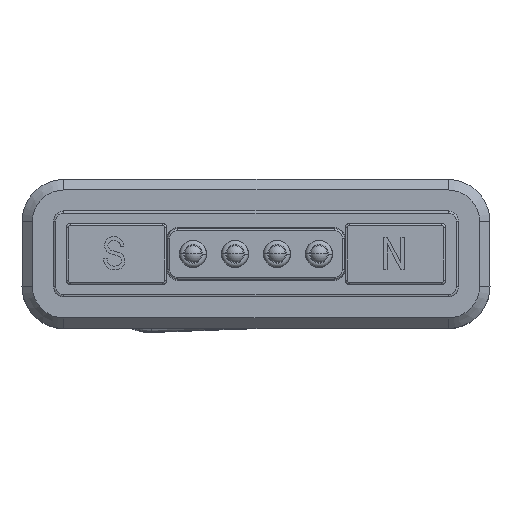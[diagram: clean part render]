
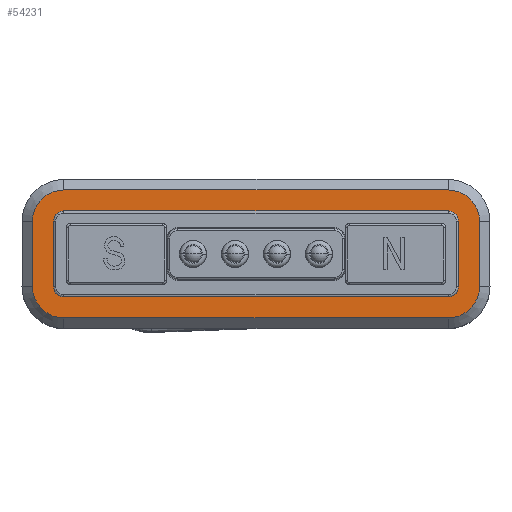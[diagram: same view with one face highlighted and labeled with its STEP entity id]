
A CAD part, top view. The second image highlights one B-rep face of the part: STEP entity #54231.
In plain terms, the highlighted planar face has unit normal (0, 0, 1).
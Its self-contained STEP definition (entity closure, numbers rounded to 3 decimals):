
#741 = AXIS2_PLACEMENT_3D ( 'NONE', #9683, #37258, #10805 ) ;
#1030 = CARTESIAN_POINT ( 'NONE',  ( -10.65, -1.55, -0.5 ) ) ;
#1350 = ORIENTED_EDGE ( 'NONE', *, *, #19401, .F. ) ;
#1521 = DIRECTION ( 'NONE',  ( 0., 0., -1. ) ) ;
#2647 = DIRECTION ( 'NONE',  ( 0., 1., 0. ) ) ;
#2835 = ORIENTED_EDGE ( 'NONE', *, *, #43955, .T. ) ;
#3294 = EDGE_CURVE ( 'NONE', #37424, #54211, #42026, .T. ) ;
#3848 = CIRCLE ( 'NONE', #7521, 1.5 ) ;
#4217 = VECTOR ( 'NONE', #20566, 1000. ) ;
#5425 = CARTESIAN_POINT ( 'NONE',  ( -9.65, -1.55, -0.5 ) ) ;
#5600 = DIRECTION ( 'NONE',  ( 0., 1., 0. ) ) ;
#5861 = DIRECTION ( 'NONE',  ( 0., 0., -1. ) ) ;
#5863 = VERTEX_POINT ( 'NONE', #23645 ) ;
#6089 = DIRECTION ( 'NONE',  ( 0., 0., -1. ) ) ;
#6376 = CARTESIAN_POINT ( 'NONE',  ( 9.15, -1.55, -0.5 ) ) ;
#6567 = ORIENTED_EDGE ( 'NONE', *, *, #45096, .F. ) ;
#6607 = VERTEX_POINT ( 'NONE', #5425 ) ;
#6695 = CIRCLE ( 'NONE', #25925, 0.5 ) ;
#6750 = CIRCLE ( 'NONE', #46231, 0.5 ) ;
#6774 = CIRCLE ( 'NONE', #22342, 1.5 ) ;
#7424 = CARTESIAN_POINT ( 'NONE',  ( -9.15, 3.05, -0.5 ) ) ;
#7521 = AXIS2_PLACEMENT_3D ( 'NONE', #19333, #36062, #5600 ) ;
#8927 = LINE ( 'NONE', #26409, #50702 ) ;
#9656 = CARTESIAN_POINT ( 'NONE',  ( -9.15, -2.05, -0.5 ) ) ;
#9683 = CARTESIAN_POINT ( 'NONE',  ( 0., 0., -0.5 ) ) ;
#10805 = DIRECTION ( 'NONE',  ( 1., 0., 0. ) ) ;
#11178 = DIRECTION ( 'NONE',  ( 0., -1., 0. ) ) ;
#11232 = EDGE_CURVE ( 'NONE', #11741, #42800, #41487, .T. ) ;
#11365 = CARTESIAN_POINT ( 'NONE',  ( 10.65, 1.55, -0.5 ) ) ;
#11433 = DIRECTION ( 'NONE',  ( 1., 0., 0. ) ) ;
#11741 = VERTEX_POINT ( 'NONE', #11365 ) ;
#11867 = DIRECTION ( 'NONE',  ( 0., 0., 1. ) ) ;
#12131 = AXIS2_PLACEMENT_3D ( 'NONE', #43207, #11867, #51248 ) ;
#12845 = VECTOR ( 'NONE', #36100, 1000. ) ;
#12846 = CARTESIAN_POINT ( 'NONE',  ( 9.15, -3.05, -0.5 ) ) ;
#12920 = ORIENTED_EDGE ( 'NONE', *, *, #42680, .T. ) ;
#12980 = CARTESIAN_POINT ( 'NONE',  ( -10.65, 1.55, -0.5 ) ) ;
#14417 = EDGE_CURVE ( 'NONE', #39064, #35145, #6750, .T. ) ;
#14710 = DIRECTION ( 'NONE',  ( -1., 0., 0. ) ) ;
#15049 = CIRCLE ( 'NONE', #26985, 0.5 ) ;
#15446 = LINE ( 'NONE', #51396, #35349 ) ;
#15477 = DIRECTION ( 'NONE',  ( 0., 0., 1. ) ) ;
#15517 = ORIENTED_EDGE ( 'NONE', *, *, #45349, .F. ) ;
#16458 = CARTESIAN_POINT ( 'NONE',  ( 9.15, 3.05, -0.5 ) ) ;
#16948 = DIRECTION ( 'NONE',  ( 0., -1., 0. ) ) ;
#16965 = VECTOR ( 'NONE', #43349, 1000. ) ;
#17939 = AXIS2_PLACEMENT_3D ( 'NONE', #40098, #5861, #27656 ) ;
#18100 = DIRECTION ( 'NONE',  ( -1., 0., 0. ) ) ;
#18328 = EDGE_LOOP ( 'NONE', ( #38152, #49532, #15517, #2835, #1350, #30088, #6567, #12920 ) ) ;
#18945 = CARTESIAN_POINT ( 'NONE',  ( -9.15, -2.05, -0.5 ) ) ;
#19059 = AXIS2_PLACEMENT_3D ( 'NONE', #26972, #45114, #18100 ) ;
#19333 = CARTESIAN_POINT ( 'NONE',  ( -9.15, 1.55, -0.5 ) ) ;
#19401 = EDGE_CURVE ( 'NONE', #11741, #5863, #43627, .T. ) ;
#19485 = VERTEX_POINT ( 'NONE', #39598 ) ;
#20566 = DIRECTION ( 'NONE',  ( 0., -1., 0. ) ) ;
#21087 = CARTESIAN_POINT ( 'NONE',  ( -9.15, 2.05, -0.5 ) ) ;
#21243 = EDGE_LOOP ( 'NONE', ( #50930, #36769, #32887, #30159, #35294, #39664, #36123, #38819 ) ) ;
#22342 = AXIS2_PLACEMENT_3D ( 'NONE', #54898, #15477, #11178 ) ;
#22556 = PLANE ( 'NONE',  #741 ) ;
#22831 = FACE_OUTER_BOUND ( 'NONE', #18328, .T. ) ;
#23645 = CARTESIAN_POINT ( 'NONE',  ( 10.65, -1.55, -0.5 ) ) ;
#23890 = CARTESIAN_POINT ( 'NONE',  ( -9.15, -3.05, -0.5 ) ) ;
#24522 = EDGE_CURVE ( 'NONE', #39064, #6607, #25183, .T. ) ;
#25183 = LINE ( 'NONE', #55174, #42379 ) ;
#25925 = AXIS2_PLACEMENT_3D ( 'NONE', #6376, #1521, #30615 ) ;
#26409 = CARTESIAN_POINT ( 'NONE',  ( -10.65, 1.55, -0.5 ) ) ;
#26413 = EDGE_CURVE ( 'NONE', #19485, #35145, #46057, .T. ) ;
#26972 = CARTESIAN_POINT ( 'NONE',  ( -9.15, -1.55, -0.5 ) ) ;
#26985 = AXIS2_PLACEMENT_3D ( 'NONE', #45451, #6089, #31964 ) ;
#27656 = DIRECTION ( 'NONE',  ( 0., 1., 0. ) ) ;
#29345 = DIRECTION ( 'NONE',  ( 0., 0., -1. ) ) ;
#29415 = EDGE_CURVE ( 'NONE', #35262, #46931, #55821, .T. ) ;
#30088 = ORIENTED_EDGE ( 'NONE', *, *, #11232, .T. ) ;
#30159 = ORIENTED_EDGE ( 'NONE', *, *, #26413, .F. ) ;
#30483 = CARTESIAN_POINT ( 'NONE',  ( 9.65, -1.55, -0.5 ) ) ;
#30615 = DIRECTION ( 'NONE',  ( 1., 0., 0. ) ) ;
#31964 = DIRECTION ( 'NONE',  ( 0., -1., 0. ) ) ;
#32887 = ORIENTED_EDGE ( 'NONE', *, *, #14417, .T. ) ;
#33658 = VECTOR ( 'NONE', #2647, 1000. ) ;
#33937 = CARTESIAN_POINT ( 'NONE',  ( 9.15, -3.05, -0.5 ) ) ;
#34434 = LINE ( 'NONE', #12846, #16965 ) ;
#35145 = VERTEX_POINT ( 'NONE', #21087 ) ;
#35262 = VERTEX_POINT ( 'NONE', #1030 ) ;
#35294 = ORIENTED_EDGE ( 'NONE', *, *, #45796, .T. ) ;
#35349 = VECTOR ( 'NONE', #11433, 1000. ) ;
#35568 = CARTESIAN_POINT ( 'NONE',  ( 9.65, 1.55, -0.5 ) ) ;
#36062 = DIRECTION ( 'NONE',  ( 0., 0., 1. ) ) ;
#36100 = DIRECTION ( 'NONE',  ( 1., 0., 0. ) ) ;
#36123 = ORIENTED_EDGE ( 'NONE', *, *, #43632, .T. ) ;
#36769 = ORIENTED_EDGE ( 'NONE', *, *, #24522, .F. ) ;
#37258 = DIRECTION ( 'NONE',  ( 0., 0., 1. ) ) ;
#37424 = VERTEX_POINT ( 'NONE', #30483 ) ;
#38152 = ORIENTED_EDGE ( 'NONE', *, *, #43210, .T. ) ;
#38358 = VERTEX_POINT ( 'NONE', #18945 ) ;
#38819 = ORIENTED_EDGE ( 'NONE', *, *, #40412, .F. ) ;
#39064 = VERTEX_POINT ( 'NONE', #41227 ) ;
#39327 = CARTESIAN_POINT ( 'NONE',  ( 10.65, 1.55, -0.5 ) ) ;
#39598 = CARTESIAN_POINT ( 'NONE',  ( 9.15, 2.05, -0.5 ) ) ;
#39664 = ORIENTED_EDGE ( 'NONE', *, *, #3294, .F. ) ;
#39927 = VERTEX_POINT ( 'NONE', #33937 ) ;
#40098 = CARTESIAN_POINT ( 'NONE',  ( 9.15, 1.55, -0.5 ) ) ;
#40412 = EDGE_CURVE ( 'NONE', #38358, #52017, #49038, .T. ) ;
#40767 = VERTEX_POINT ( 'NONE', #12980 ) ;
#41227 = CARTESIAN_POINT ( 'NONE',  ( -9.65, 1.55, -0.5 ) ) ;
#41487 = CIRCLE ( 'NONE', #12131, 1.5 ) ;
#42026 = LINE ( 'NONE', #45460, #33658 ) ;
#42379 = VECTOR ( 'NONE', #56020, 1000. ) ;
#42680 = EDGE_CURVE ( 'NONE', #45193, #40767, #3848, .T. ) ;
#42770 = CIRCLE ( 'NONE', #17939, 0.5 ) ;
#42800 = VERTEX_POINT ( 'NONE', #16458 ) ;
#43207 = CARTESIAN_POINT ( 'NONE',  ( 9.15, 1.55, -0.5 ) ) ;
#43210 = EDGE_CURVE ( 'NONE', #40767, #35262, #8927, .T. ) ;
#43349 = DIRECTION ( 'NONE',  ( -1., 0., 0. ) ) ;
#43627 = LINE ( 'NONE', #39327, #4217 ) ;
#43632 = EDGE_CURVE ( 'NONE', #37424, #52017, #6695, .T. ) ;
#43954 = CARTESIAN_POINT ( 'NONE',  ( 9.15, -2.05, -0.5 ) ) ;
#43955 = EDGE_CURVE ( 'NONE', #39927, #5863, #6774, .T. ) ;
#45096 = EDGE_CURVE ( 'NONE', #45193, #42800, #15446, .T. ) ;
#45114 = DIRECTION ( 'NONE',  ( 0., 0., 1. ) ) ;
#45193 = VERTEX_POINT ( 'NONE', #7424 ) ;
#45349 = EDGE_CURVE ( 'NONE', #39927, #46931, #34434, .T. ) ;
#45451 = CARTESIAN_POINT ( 'NONE',  ( -9.15, -1.55, -0.5 ) ) ;
#45460 = CARTESIAN_POINT ( 'NONE',  ( 9.65, -1.55, -0.5 ) ) ;
#45796 = EDGE_CURVE ( 'NONE', #19485, #54211, #42770, .T. ) ;
#46057 = LINE ( 'NONE', #54692, #49966 ) ;
#46231 = AXIS2_PLACEMENT_3D ( 'NONE', #50936, #29345, #55259 ) ;
#46931 = VERTEX_POINT ( 'NONE', #23890 ) ;
#47165 = EDGE_CURVE ( 'NONE', #38358, #6607, #15049, .T. ) ;
#49038 = LINE ( 'NONE', #9656, #12845 ) ;
#49532 = ORIENTED_EDGE ( 'NONE', *, *, #29415, .T. ) ;
#49966 = VECTOR ( 'NONE', #14710, 1000. ) ;
#50702 = VECTOR ( 'NONE', #16948, 1000. ) ;
#50930 = ORIENTED_EDGE ( 'NONE', *, *, #47165, .T. ) ;
#50936 = CARTESIAN_POINT ( 'NONE',  ( -9.15, 1.55, -0.5 ) ) ;
#51248 = DIRECTION ( 'NONE',  ( 1., 0., 0. ) ) ;
#51396 = CARTESIAN_POINT ( 'NONE',  ( -9.15, 3.05, -0.5 ) ) ;
#52017 = VERTEX_POINT ( 'NONE', #43954 ) ;
#53085 = FACE_BOUND ( 'NONE', #21243, .T. ) ;
#54211 = VERTEX_POINT ( 'NONE', #35568 ) ;
#54231 = ADVANCED_FACE ( 'NONE', ( #22831, #53085 ), #22556, .T. ) ;
#54692 = CARTESIAN_POINT ( 'NONE',  ( 9.15, 2.05, -0.5 ) ) ;
#54898 = CARTESIAN_POINT ( 'NONE',  ( 9.15, -1.55, -0.5 ) ) ;
#55174 = CARTESIAN_POINT ( 'NONE',  ( -9.65, 1.55, -0.5 ) ) ;
#55259 = DIRECTION ( 'NONE',  ( -1., 0., 0. ) ) ;
#55821 = CIRCLE ( 'NONE', #19059, 1.5 ) ;
#56020 = DIRECTION ( 'NONE',  ( 0., -1., 0. ) ) ;
